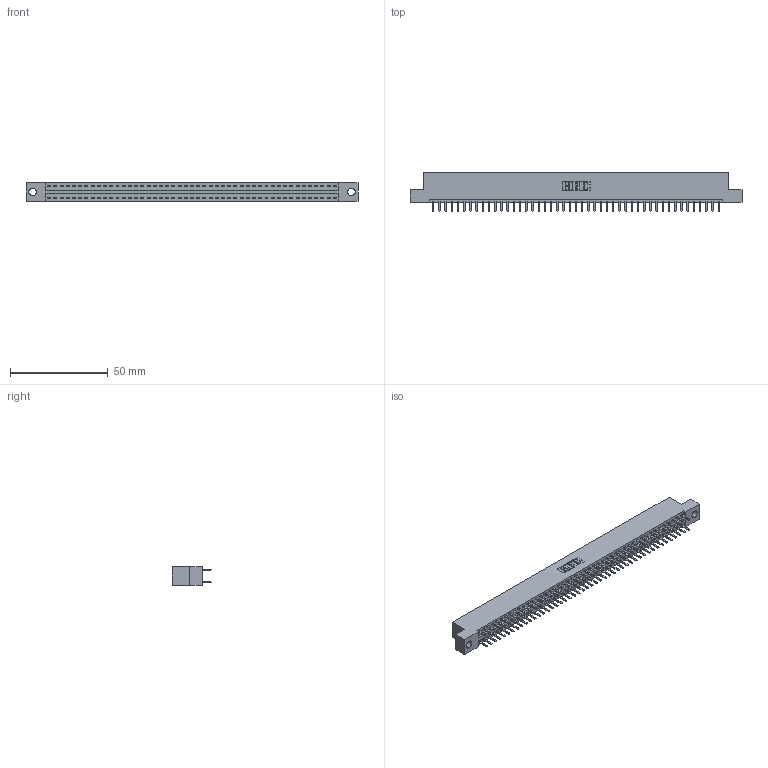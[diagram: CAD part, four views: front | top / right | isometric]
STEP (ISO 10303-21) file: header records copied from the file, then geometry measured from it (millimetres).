
FILE_DESCRIPTION (( 'STEP AP203' ), '1' );
FILE_NAME ('396-094-520-204.STEP', '2018-09-12T11:56:44', ( '' ), ( '' ), 'SwSTEP 2.0', 'SolidWorks 2016', '' );
FILE_SCHEMA (( 'CONFIG_CONTROL_DESIGN' ));
Length unit declared in the file: inch
Products named in the file (3): 396-094-520-204; 346 Part_Flush Mounting Lugs - 0.156 Dia-TH; 345-292-001_345-293-120
Assembly tree (95 placements, depth 2):
  396-094-520-204
    346 Part_Flush Mounting Lugs - 0.156 Dia-TH
    345-292-001_345-293-120  x94
Bounding box: 169.8 x 20.02 x 9.4 mm (x, y, z)
Volume: 16467.2 mm3; surface area: 22430.3 mm2
Topology: 95 solids, 95 shells, 5386 faces, 15651 edges, 10182 vertices
Faces by surface type: plane 3554, cylinder 1832
Entity records: 30117 total; most frequent: CARTESIAN_POINT 4968, ORIENTED_EDGE 4890, DIRECTION 4417, EDGE_CURVE 2445, LINE 2121, VECTOR 2121, VERTEX_POINT 1626, AXIS2_PLACEMENT_3D 1148
